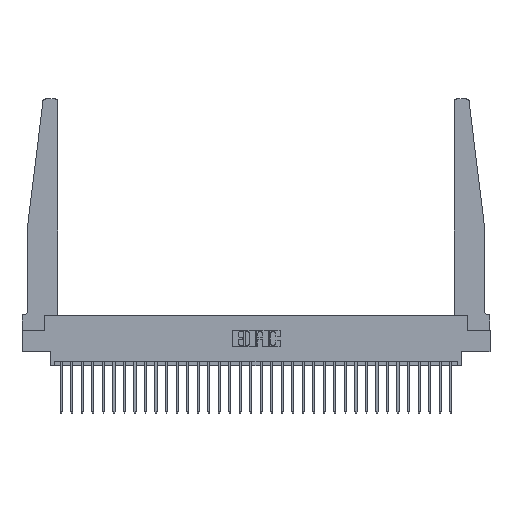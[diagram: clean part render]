
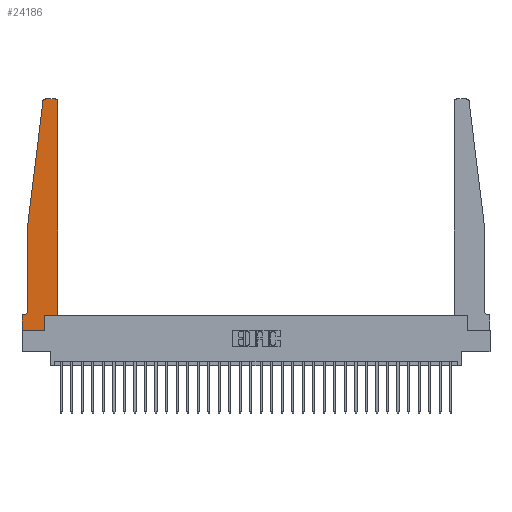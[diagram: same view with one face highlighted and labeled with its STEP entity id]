
A CAD part, top view. The second image highlights one B-rep face of the part: STEP entity #24186.
In plain terms, the highlighted planar face has unit normal (0, 0, 1).
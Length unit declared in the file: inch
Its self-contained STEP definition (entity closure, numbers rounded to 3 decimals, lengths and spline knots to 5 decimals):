
#114 = CIRCLE ( 'NONE', #7548, 0.03 ) ;
#286 = CARTESIAN_POINT ( 'NONE',  ( 0.27653, 2.75, 0.37 ) ) ;
#478 = DIRECTION ( 'NONE',  ( 1., 0., 0. ) ) ;
#523 = VERTEX_POINT ( 'NONE', #10851 ) ;
#567 = VERTEX_POINT ( 'NONE', #24560 ) ;
#574 = DIRECTION ( 'NONE',  ( -1., 0., 0. ) ) ;
#778 = PLANE ( 'NONE',  #19301 ) ;
#926 = CARTESIAN_POINT ( 'NONE',  ( 0.065, 1.25, 0.37 ) ) ;
#940 = EDGE_CURVE ( 'NONE', #567, #17549, #22200, .T. ) ;
#1970 = VECTOR ( 'NONE', #24006, 39.37008 ) ;
#1988 = AXIS2_PLACEMENT_3D ( 'NONE', #6307, #15778, #23720 ) ;
#3116 = DIRECTION ( 'NONE',  ( 0., 0., 1. ) ) ;
#3638 = LINE ( 'NONE', #23074, #16190 ) ;
#3888 = CARTESIAN_POINT ( 'NONE',  ( 0.425, 0.18, 0.37 ) ) ;
#3966 = VECTOR ( 'NONE', #11002, 39.37008 ) ;
#3984 = CARTESIAN_POINT ( 'NONE',  ( 0.015, 0.1875, 0.37 ) ) ;
#4545 = ORIENTED_EDGE ( 'NONE', *, *, #22268, .T. ) ;
#4919 = CARTESIAN_POINT ( 'NONE',  ( 0.065, 1.25, 0.37 ) ) ;
#4954 = CARTESIAN_POINT ( 'NONE',  ( 0.25, 2.75, 0.37 ) ) ;
#5146 = VERTEX_POINT ( 'NONE', #3984 ) ;
#5294 = LINE ( 'NONE', #926, #18556 ) ;
#5516 = ORIENTED_EDGE ( 'NONE', *, *, #30407, .T. ) ;
#5683 = CARTESIAN_POINT ( 'NONE',  ( 0.27653, 2.72, 0.37 ) ) ;
#5916 = DIRECTION ( 'NONE',  ( 0., 0., 1. ) ) ;
#6307 = CARTESIAN_POINT ( 'NONE',  ( 0.015, 0.2375, 0.37 ) ) ;
#6618 = DIRECTION ( 'NONE',  ( 0., -1., 0. ) ) ;
#7548 = AXIS2_PLACEMENT_3D ( 'NONE', #5683, #27602, #20291 ) ;
#7648 = VERTEX_POINT ( 'NONE', #30611 ) ;
#7716 = CARTESIAN_POINT ( 'NONE',  ( 0.425, 0.18, 0.37 ) ) ;
#7836 = EDGE_CURVE ( 'NONE', #26379, #23327, #24372, .T. ) ;
#8524 = EDGE_CURVE ( 'NONE', #15418, #523, #5294, .T. ) ;
#8670 = VERTEX_POINT ( 'NONE', #3888 ) ;
#8739 = VERTEX_POINT ( 'NONE', #28130 ) ;
#9122 = VECTOR ( 'NONE', #6618, 39.37008 ) ;
#9246 = LINE ( 'NONE', #4919, #9122 ) ;
#9301 = EDGE_CURVE ( 'NONE', #523, #7648, #9246, .T. ) ;
#9826 = LINE ( 'NONE', #17300, #1970 ) ;
#9829 = ORIENTED_EDGE ( 'NONE', *, *, #30508, .T. ) ;
#10851 = CARTESIAN_POINT ( 'NONE',  ( 0.065, 1.25, 0.37 ) ) ;
#10952 = ORIENTED_EDGE ( 'NONE', *, *, #29816, .T. ) ;
#11002 = DIRECTION ( 'NONE',  ( 0., -1., 0. ) ) ;
#11535 = ORIENTED_EDGE ( 'NONE', *, *, #25527, .T. ) ;
#11700 = ORIENTED_EDGE ( 'NONE', *, *, #8524, .T. ) ;
#12312 = VERTEX_POINT ( 'NONE', #15580 ) ;
#12429 = EDGE_CURVE ( 'NONE', #5146, #21641, #3638, .T. ) ;
#12895 = CARTESIAN_POINT ( 'NONE',  ( 0., 0.1875, 0.37 ) ) ;
#14333 = ORIENTED_EDGE ( 'NONE', *, *, #940, .T. ) ;
#14570 = LINE ( 'NONE', #7716, #18959 ) ;
#15016 = DIRECTION ( 'NONE',  ( 1., 0., 0. ) ) ;
#15418 = VERTEX_POINT ( 'NONE', #23230 ) ;
#15516 = VECTOR ( 'NONE', #574, 39.37008 ) ;
#15580 = CARTESIAN_POINT ( 'NONE',  ( 0.2605, 0.18, 0.37 ) ) ;
#15778 = DIRECTION ( 'NONE',  ( 0., 0., -1. ) ) ;
#16190 = VECTOR ( 'NONE', #18406, 39.37008 ) ;
#16979 = ORIENTED_EDGE ( 'NONE', *, *, #12429, .T. ) ;
#17215 = CIRCLE ( 'NONE', #30139, 0.03 ) ;
#17300 = CARTESIAN_POINT ( 'NONE',  ( 0.2605, 0.18, 0.37 ) ) ;
#17549 = VERTEX_POINT ( 'NONE', #25355 ) ;
#18308 = CARTESIAN_POINT ( 'NONE',  ( 0.395, 2.72, 0.37 ) ) ;
#18361 = EDGE_LOOP ( 'NONE', ( #26227, #5516, #11700, #23174, #23563, #16979, #18656, #14333, #11535, #10952, #9829, #4545 ) ) ;
#18406 = DIRECTION ( 'NONE',  ( -1., 0., 0. ) ) ;
#18425 = CARTESIAN_POINT ( 'NONE',  ( 0.425, 0.18, 0.37 ) ) ;
#18556 = VECTOR ( 'NONE', #19752, 39.37008 ) ;
#18656 = ORIENTED_EDGE ( 'NONE', *, *, #27068, .T. ) ;
#18877 = LINE ( 'NONE', #18425, #27424 ) ;
#18959 = VECTOR ( 'NONE', #26869, 39.37008 ) ;
#19301 = AXIS2_PLACEMENT_3D ( 'NONE', #12895, #5916, #478 ) ;
#19752 = DIRECTION ( 'NONE',  ( -0.122, -0.992, 0. ) ) ;
#19984 = EDGE_CURVE ( 'NONE', #7648, #5146, #26821, .T. ) ;
#20291 = DIRECTION ( 'NONE',  ( 1., 0., 0. ) ) ;
#20753 = DIRECTION ( 'NONE',  ( 0., 1., 0. ) ) ;
#21641 = VERTEX_POINT ( 'NONE', #25417 ) ;
#22113 = FACE_OUTER_BOUND ( 'NONE', #18361, .T. ) ;
#22200 = LINE ( 'NONE', #24970, #30033 ) ;
#22268 = EDGE_CURVE ( 'NONE', #8739, #26379, #17215, .T. ) ;
#22707 = LINE ( 'NONE', #29529, #3966 ) ;
#23074 = CARTESIAN_POINT ( 'NONE',  ( 0.065, 0.1875, 0.37 ) ) ;
#23174 = ORIENTED_EDGE ( 'NONE', *, *, #9301, .T. ) ;
#23230 = CARTESIAN_POINT ( 'NONE',  ( 0.24675, 2.72367, 0.37 ) ) ;
#23327 = VERTEX_POINT ( 'NONE', #286 ) ;
#23563 = ORIENTED_EDGE ( 'NONE', *, *, #19984, .T. ) ;
#23720 = DIRECTION ( 'NONE',  ( -1., 0., 0. ) ) ;
#24006 = DIRECTION ( 'NONE',  ( 0., 1., 0. ) ) ;
#24186 = ADVANCED_FACE ( 'NONE', ( #22113 ), #778, .T. ) ;
#24372 = LINE ( 'NONE', #4954, #15516 ) ;
#24560 = CARTESIAN_POINT ( 'NONE',  ( 0., 0., 0.37 ) ) ;
#24724 = DIRECTION ( 'NONE',  ( 1., 0., 0. ) ) ;
#24970 = CARTESIAN_POINT ( 'NONE',  ( 0., 0., 0.37 ) ) ;
#25355 = CARTESIAN_POINT ( 'NONE',  ( 0.2605, 0., 0.37 ) ) ;
#25417 = CARTESIAN_POINT ( 'NONE',  ( 0., 0.1875, 0.37 ) ) ;
#25527 = EDGE_CURVE ( 'NONE', #17549, #12312, #9826, .T. ) ;
#26227 = ORIENTED_EDGE ( 'NONE', *, *, #7836, .T. ) ;
#26379 = VERTEX_POINT ( 'NONE', #29183 ) ;
#26821 = CIRCLE ( 'NONE', #1988, 0.05 ) ;
#26869 = DIRECTION ( 'NONE',  ( 1., 0., 0. ) ) ;
#27068 = EDGE_CURVE ( 'NONE', #21641, #567, #22707, .T. ) ;
#27424 = VECTOR ( 'NONE', #20753, 39.37008 ) ;
#27602 = DIRECTION ( 'NONE',  ( 0., 0., 1. ) ) ;
#28130 = CARTESIAN_POINT ( 'NONE',  ( 0.425, 2.72, 0.37 ) ) ;
#29183 = CARTESIAN_POINT ( 'NONE',  ( 0.395, 2.75, 0.37 ) ) ;
#29529 = CARTESIAN_POINT ( 'NONE',  ( 0., 0., 0.37 ) ) ;
#29816 = EDGE_CURVE ( 'NONE', #12312, #8670, #14570, .T. ) ;
#30033 = VECTOR ( 'NONE', #15016, 39.37008 ) ;
#30139 = AXIS2_PLACEMENT_3D ( 'NONE', #18308, #3116, #24724 ) ;
#30407 = EDGE_CURVE ( 'NONE', #23327, #15418, #114, .T. ) ;
#30508 = EDGE_CURVE ( 'NONE', #8670, #8739, #18877, .T. ) ;
#30611 = CARTESIAN_POINT ( 'NONE',  ( 0.065, 0.2375, 0.37 ) ) ;
